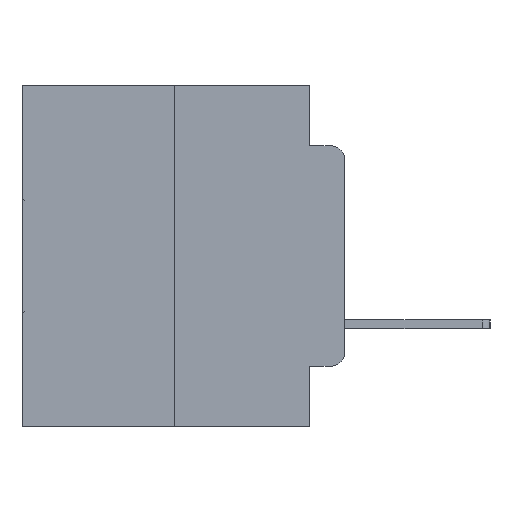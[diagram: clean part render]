
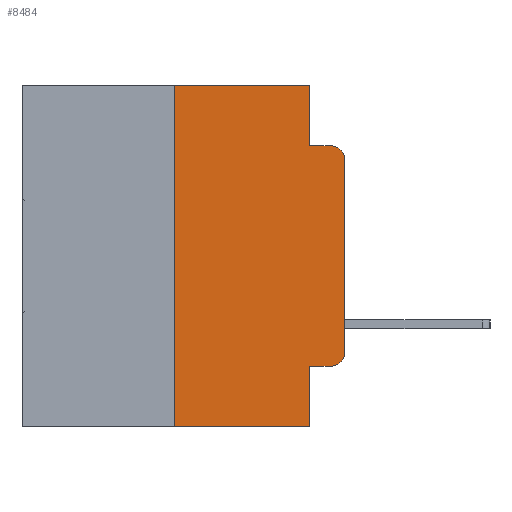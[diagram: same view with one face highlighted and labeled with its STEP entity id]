
A CAD part, left-side view. The second image highlights one B-rep face of the part: STEP entity #8484.
In plain terms, the highlighted planar face has unit normal (-1, 0, 0).
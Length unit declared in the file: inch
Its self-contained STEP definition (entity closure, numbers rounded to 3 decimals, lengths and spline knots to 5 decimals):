
#155 = LINE ( 'NONE', #13437, #23310 ) ;
#1053 = PLANE ( 'NONE',  #21779 ) ;
#1502 = ORIENTED_EDGE ( 'NONE', *, *, #20211, .F. ) ;
#1818 = FACE_OUTER_BOUND ( 'NONE', #11398, .T. ) ;
#3100 = DIRECTION ( 'NONE',  ( 0., 0., -1. ) ) ;
#3369 = DIRECTION ( 'NONE',  ( 1., 0., 0. ) ) ;
#4072 = CARTESIAN_POINT ( 'NONE',  ( 0., 0.25, -0.5 ) ) ;
#4168 = VERTEX_POINT ( 'NONE', #10499 ) ;
#5005 = VECTOR ( 'NONE', #13344, 39.37008 ) ;
#5380 = DIRECTION ( 'NONE',  ( -1., 0., 0. ) ) ;
#5597 = AXIS2_PLACEMENT_3D ( 'NONE', #25476, #12410, #27651 ) ;
#5667 = VERTEX_POINT ( 'NONE', #13327 ) ;
#5960 = VECTOR ( 'NONE', #18419, 39.37008 ) ;
#6771 = ORIENTED_EDGE ( 'NONE', *, *, #15837, .F. ) ;
#7059 = VERTEX_POINT ( 'NONE', #20598 ) ;
#8484 = ADVANCED_FACE ( 'NONE', ( #1818 ), #1053, .F. ) ;
#8835 = LINE ( 'NONE', #11439, #26323 ) ;
#8853 = VERTEX_POINT ( 'NONE', #19965 ) ;
#9653 = ORIENTED_EDGE ( 'NONE', *, *, #14354, .F. ) ;
#9859 = ORIENTED_EDGE ( 'NONE', *, *, #17311, .F. ) ;
#9898 = EDGE_CURVE ( 'NONE', #20286, #8853, #11755, .T. ) ;
#10175 = LINE ( 'NONE', #15735, #21169 ) ;
#10247 = CARTESIAN_POINT ( 'NONE',  ( 0., 0.473, 0. ) ) ;
#10499 = CARTESIAN_POINT ( 'NONE',  ( 0., 0., -0.1085 ) ) ;
#10503 = VECTOR ( 'NONE', #3100, 39.37008 ) ;
#10679 = ORIENTED_EDGE ( 'NONE', *, *, #12856, .T. ) ;
#10960 = CARTESIAN_POINT ( 'NONE',  ( 0., 0.25, 0. ) ) ;
#11049 = DIRECTION ( 'NONE',  ( 0., 0., 1. ) ) ;
#11167 = DIRECTION ( 'NONE',  ( 0., -1., 0. ) ) ;
#11398 = EDGE_LOOP ( 'NONE', ( #12192, #16967, #1502, #9859, #19805, #6771, #23704, #9653, #10679, #19453 ) ) ;
#11439 = CARTESIAN_POINT ( 'NONE',  ( 0., 0.051, -0.4115 ) ) ;
#11480 = VECTOR ( 'NONE', #11167, 39.37008 ) ;
#11579 = EDGE_CURVE ( 'NONE', #5667, #7059, #155, .T. ) ;
#11755 = CIRCLE ( 'NONE', #5597, 0.02 ) ;
#11956 = LINE ( 'NONE', #27020, #5960 ) ;
#11967 = VERTEX_POINT ( 'NONE', #23353 ) ;
#12192 = ORIENTED_EDGE ( 'NONE', *, *, #23120, .T. ) ;
#12410 = DIRECTION ( 'NONE',  ( -1., 0., 0. ) ) ;
#12856 = EDGE_CURVE ( 'NONE', #13745, #20286, #8835, .T. ) ;
#13327 = CARTESIAN_POINT ( 'NONE',  ( 0., 0.25, 0. ) ) ;
#13344 = DIRECTION ( 'NONE',  ( 0., -1., 0. ) ) ;
#13437 = CARTESIAN_POINT ( 'NONE',  ( 0., 0.473, 0. ) ) ;
#13729 = VECTOR ( 'NONE', #11049, 39.37008 ) ;
#13745 = VERTEX_POINT ( 'NONE', #23355 ) ;
#14354 = EDGE_CURVE ( 'NONE', #13745, #27422, #17084, .T. ) ;
#15735 = CARTESIAN_POINT ( 'NONE',  ( 0., 0.051, 0. ) ) ;
#15768 = CARTESIAN_POINT ( 'NONE',  ( 0., 0.02, -0.4115 ) ) ;
#15837 = EDGE_CURVE ( 'NONE', #19542, #5667, #19554, .T. ) ;
#16268 = LINE ( 'NONE', #26396, #5005 ) ;
#16673 = CARTESIAN_POINT ( 'NONE',  ( 0., 0.051, 0. ) ) ;
#16967 = ORIENTED_EDGE ( 'NONE', *, *, #21690, .T. ) ;
#17084 = LINE ( 'NONE', #16673, #10503 ) ;
#17311 = EDGE_CURVE ( 'NONE', #7059, #24677, #10175, .T. ) ;
#17944 = DIRECTION ( 'NONE',  ( 0., 0., -1. ) ) ;
#18004 = DIRECTION ( 'NONE',  ( 0., -1., 0. ) ) ;
#18419 = DIRECTION ( 'NONE',  ( 0., 0., 1. ) ) ;
#18743 = CARTESIAN_POINT ( 'NONE',  ( 0., 0.02, -0.1085 ) ) ;
#19095 = DIRECTION ( 'NONE',  ( 0., 0., -1. ) ) ;
#19126 = EDGE_CURVE ( 'NONE', #19542, #27422, #23129, .T. ) ;
#19453 = ORIENTED_EDGE ( 'NONE', *, *, #9898, .T. ) ;
#19542 = VERTEX_POINT ( 'NONE', #4072 ) ;
#19554 = LINE ( 'NONE', #10960, #13729 ) ;
#19805 = ORIENTED_EDGE ( 'NONE', *, *, #11579, .F. ) ;
#19965 = CARTESIAN_POINT ( 'NONE',  ( 0., 0., -0.3915 ) ) ;
#20211 = EDGE_CURVE ( 'NONE', #24677, #11967, #16268, .T. ) ;
#20286 = VERTEX_POINT ( 'NONE', #15768 ) ;
#20598 = CARTESIAN_POINT ( 'NONE',  ( 0., 0.051, 0. ) ) ;
#20691 = CARTESIAN_POINT ( 'NONE',  ( 0., 0.051, -0.5 ) ) ;
#20948 = DIRECTION ( 'NONE',  ( 0., 0., -1. ) ) ;
#21169 = VECTOR ( 'NONE', #17944, 39.37008 ) ;
#21690 = EDGE_CURVE ( 'NONE', #4168, #11967, #22324, .T. ) ;
#21779 = AXIS2_PLACEMENT_3D ( 'NONE', #10247, #3369, #19095 ) ;
#22324 = CIRCLE ( 'NONE', #26973, 0.02 ) ;
#23120 = EDGE_CURVE ( 'NONE', #8853, #4168, #11956, .T. ) ;
#23129 = LINE ( 'NONE', #28528, #11480 ) ;
#23310 = VECTOR ( 'NONE', #26481, 39.37008 ) ;
#23353 = CARTESIAN_POINT ( 'NONE',  ( 0., 0.02, -0.0885 ) ) ;
#23355 = CARTESIAN_POINT ( 'NONE',  ( 0., 0.051, -0.4115 ) ) ;
#23704 = ORIENTED_EDGE ( 'NONE', *, *, #19126, .T. ) ;
#24677 = VERTEX_POINT ( 'NONE', #28827 ) ;
#25476 = CARTESIAN_POINT ( 'NONE',  ( 0., 0.02, -0.3915 ) ) ;
#26323 = VECTOR ( 'NONE', #18004, 39.37008 ) ;
#26396 = CARTESIAN_POINT ( 'NONE',  ( 0., 0.051, -0.0885 ) ) ;
#26481 = DIRECTION ( 'NONE',  ( 0., -1., 0. ) ) ;
#26973 = AXIS2_PLACEMENT_3D ( 'NONE', #18743, #5380, #20948 ) ;
#27020 = CARTESIAN_POINT ( 'NONE',  ( 0., 0., 0. ) ) ;
#27422 = VERTEX_POINT ( 'NONE', #20691 ) ;
#27651 = DIRECTION ( 'NONE',  ( 0., 0., -1. ) ) ;
#28528 = CARTESIAN_POINT ( 'NONE',  ( 0., 0.473, -0.5 ) ) ;
#28827 = CARTESIAN_POINT ( 'NONE',  ( 0., 0.051, -0.0885 ) ) ;
